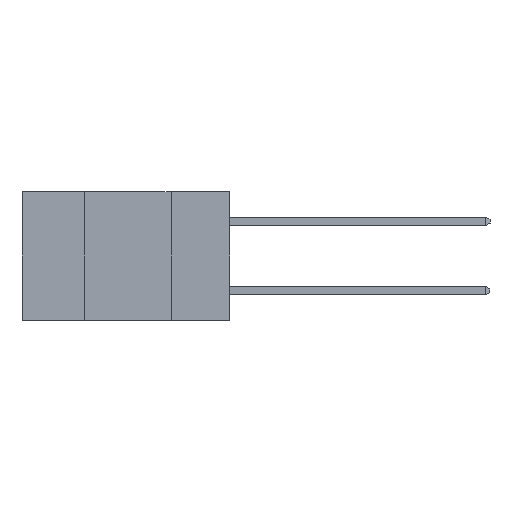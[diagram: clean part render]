
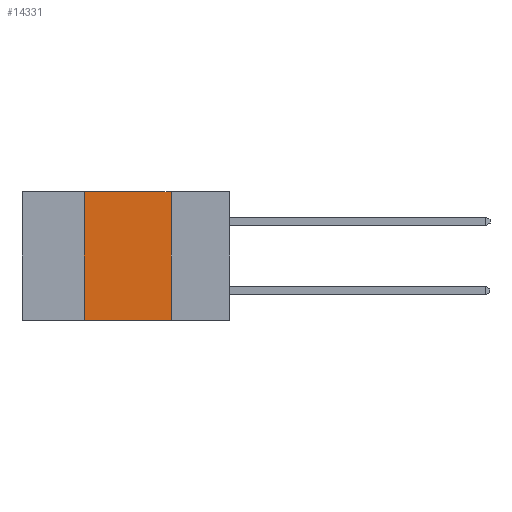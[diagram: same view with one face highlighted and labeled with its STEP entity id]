
A CAD part, left-side view. The second image highlights one B-rep face of the part: STEP entity #14331.
In plain terms, the highlighted planar face has unit normal (-1, 0, 0).
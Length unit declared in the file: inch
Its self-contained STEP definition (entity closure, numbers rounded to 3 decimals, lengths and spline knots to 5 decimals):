
#728 = EDGE_CURVE ( 'NONE', #1315, #4686, #4588, .T. ) ;
#771 = DIRECTION ( 'NONE',  ( 0., 0., -1. ) ) ;
#924 = FACE_OUTER_BOUND ( 'NONE', #6171, .T. ) ;
#1315 = VERTEX_POINT ( 'NONE', #14836 ) ;
#1761 = VECTOR ( 'NONE', #13442, 39.37008 ) ;
#1855 = DIRECTION ( 'NONE',  ( 0., -1., 0. ) ) ;
#1910 = DIRECTION ( 'NONE',  ( 1., 0., 0. ) ) ;
#3319 = VECTOR ( 'NONE', #1855, 39.37008 ) ;
#4316 = VERTEX_POINT ( 'NONE', #6316 ) ;
#4588 = LINE ( 'NONE', #7460, #1761 ) ;
#4686 = VERTEX_POINT ( 'NONE', #8244 ) ;
#5474 = EDGE_CURVE ( 'NONE', #7931, #4316, #10115, .T. ) ;
#5873 = CARTESIAN_POINT ( 'NONE',  ( 0., 0.17, 0. ) ) ;
#6171 = EDGE_LOOP ( 'NONE', ( #10033, #6853, #10413, #14021 ) ) ;
#6316 = CARTESIAN_POINT ( 'NONE',  ( 0., 0.17, 0. ) ) ;
#6805 = CARTESIAN_POINT ( 'NONE',  ( 0., 0.6, 0. ) ) ;
#6853 = ORIENTED_EDGE ( 'NONE', *, *, #5474, .F. ) ;
#7144 = VECTOR ( 'NONE', #13222, 39.37008 ) ;
#7460 = CARTESIAN_POINT ( 'NONE',  ( 0., 0.6, -0.37 ) ) ;
#7669 = CARTESIAN_POINT ( 'NONE',  ( 0., 0.42, 0. ) ) ;
#7719 = LINE ( 'NONE', #5873, #10508 ) ;
#7931 = VERTEX_POINT ( 'NONE', #7669 ) ;
#8012 = PLANE ( 'NONE',  #10950 ) ;
#8244 = CARTESIAN_POINT ( 'NONE',  ( 0., 0.17, -0.37 ) ) ;
#8622 = EDGE_CURVE ( 'NONE', #1315, #7931, #10315, .T. ) ;
#8914 = CARTESIAN_POINT ( 'NONE',  ( 0., 0.6, 0. ) ) ;
#10033 = ORIENTED_EDGE ( 'NONE', *, *, #15078, .F. ) ;
#10115 = LINE ( 'NONE', #8914, #3319 ) ;
#10315 = LINE ( 'NONE', #13266, #7144 ) ;
#10413 = ORIENTED_EDGE ( 'NONE', *, *, #8622, .F. ) ;
#10508 = VECTOR ( 'NONE', #11816, 39.37008 ) ;
#10950 = AXIS2_PLACEMENT_3D ( 'NONE', #6805, #1910, #771 ) ;
#11816 = DIRECTION ( 'NONE',  ( 0., 0., -1. ) ) ;
#13222 = DIRECTION ( 'NONE',  ( 0., 0., 1. ) ) ;
#13266 = CARTESIAN_POINT ( 'NONE',  ( 0., 0.42, 0. ) ) ;
#13442 = DIRECTION ( 'NONE',  ( 0., -1., 0. ) ) ;
#14021 = ORIENTED_EDGE ( 'NONE', *, *, #728, .T. ) ;
#14331 = ADVANCED_FACE ( 'NONE', ( #924 ), #8012, .F. ) ;
#14836 = CARTESIAN_POINT ( 'NONE',  ( 0., 0.42, -0.37 ) ) ;
#15078 = EDGE_CURVE ( 'NONE', #4316, #4686, #7719, .T. ) ;
